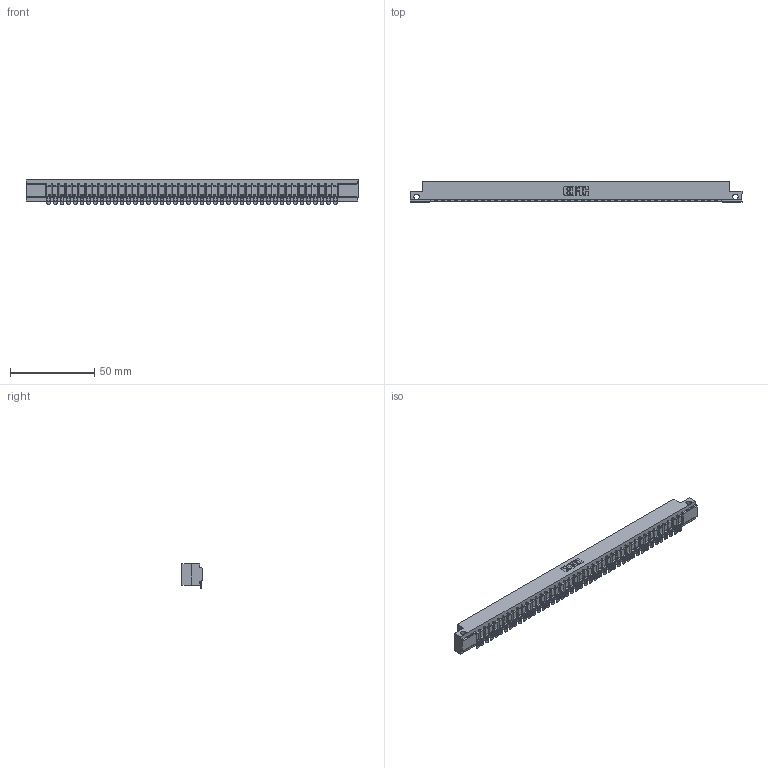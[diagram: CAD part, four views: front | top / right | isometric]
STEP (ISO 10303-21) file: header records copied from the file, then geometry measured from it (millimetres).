
FILE_DESCRIPTION (( 'STEP AP203' ), '1' );
FILE_NAME ('307-044-554-112.STEP', '2018-08-06T02:02:18', ( '' ), ( '' ), 'SwSTEP 2.0', 'SolidWorks 2016', '' );
FILE_SCHEMA (( 'CONFIG_CONTROL_DESIGN' ));
Length unit declared in the file: inch
Products named in the file (3): 307 Part_.128 Dia Side Mounting Holes; 307-290-002_554; 307-044-554-112
Assembly tree (45 placements, depth 2):
  307-044-554-112
    307 Part_.128 Dia Side Mounting Holes
    307-290-002_554  x44
Bounding box: 197.36 x 12.01 x 14.52 mm (x, y, z)
Volume: 21008.5 mm3; surface area: 26617.4 mm2
Topology: 45 solids, 45 shells, 3727 faces, 11455 edges, 7514 vertices
Faces by surface type: plane 2094, cylinder 1543, sphere 90
Entity records: 38441 total; most frequent: CARTESIAN_POINT 6486, ORIENTED_EDGE 6476, DIRECTION 6306, EDGE_CURVE 3238, LINE 2474, VECTOR 2474, VERTEX_POINT 2096, AXIS2_PLACEMENT_3D 1916
